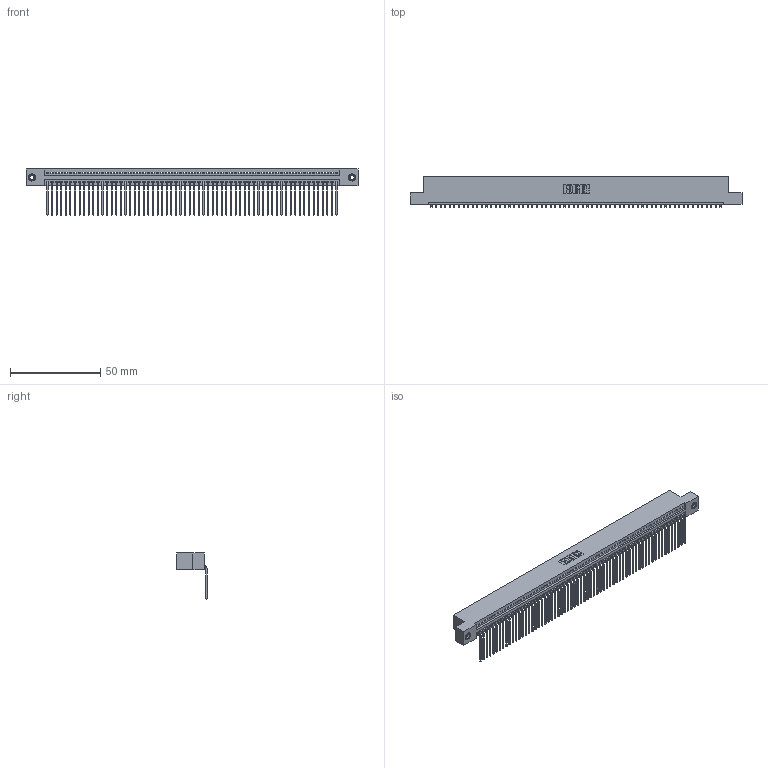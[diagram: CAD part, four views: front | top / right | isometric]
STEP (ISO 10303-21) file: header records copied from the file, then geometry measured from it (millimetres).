
FILE_DESCRIPTION (( 'STEP AP203' ), '1' );
FILE_NAME ('345-064-559-108.STEP', '2019-10-11T16:05:43', ( '' ), ( '' ), 'SwSTEP 2.0', 'SolidWorks 2016', '' );
FILE_SCHEMA (( 'CONFIG_CONTROL_DESIGN' ));
Length unit declared in the file: inch
Products named in the file (4): 345 Part_Flush Mounting Lugs - 0.156 Dia-TI; 345-064-559-108; 345-292-001_558 559 Tail - 1; 345-250-001_345-250-003-102
Assembly tree (67 placements, depth 2):
  345-064-559-108
    345 Part_Flush Mounting Lugs - 0.156 Dia-TI
    345-292-001_558 559 Tail - 1  x64
    345-250-001_345-250-003-102  x2
Bounding box: 183.77 x 16.75 x 25.53 mm (x, y, z)
Volume: 17841.5 mm3; surface area: 25280.9 mm2
Topology: 67 solids, 67 shells, 4026 faces, 12125 edges, 7990 vertices
Faces by surface type: plane 2800, cylinder 1210, cone 12, torus 4
Entity records: 46476 total; most frequent: CARTESIAN_POINT 8031, ORIENTED_EDGE 8022, DIRECTION 7009, EDGE_CURVE 4011, VECTOR 3603, LINE 3603, VERTEX_POINT 2668, AXIS2_PLACEMENT_3D 1703
